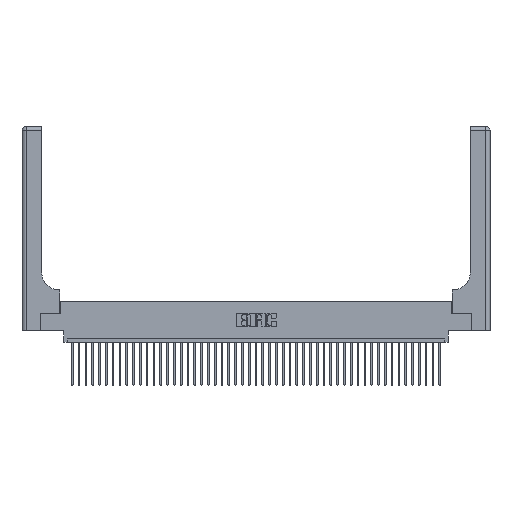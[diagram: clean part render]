
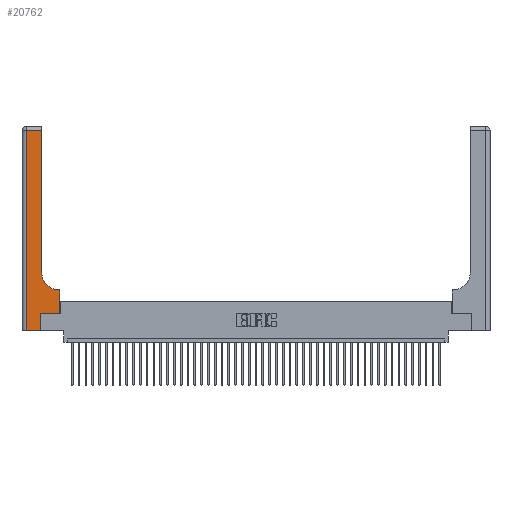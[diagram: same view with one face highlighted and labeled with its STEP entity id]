
A CAD part, top view. The second image highlights one B-rep face of the part: STEP entity #20762.
In plain terms, the highlighted planar face has unit normal (0, 0, 1).
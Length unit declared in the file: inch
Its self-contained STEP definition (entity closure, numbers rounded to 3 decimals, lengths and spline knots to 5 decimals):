
#450 = CARTESIAN_POINT ( 'NONE',  ( 0.269, 0.25, 0.37 ) ) ;
#1973 = VECTOR ( 'NONE', #14406, 39.37008 ) ;
#2352 = VERTEX_POINT ( 'NONE', #27724 ) ;
#2886 = ORIENTED_EDGE ( 'NONE', *, *, #30158, .T. ) ;
#3375 = CARTESIAN_POINT ( 'NONE',  ( 0.269, 0.25, 0.37 ) ) ;
#3590 = ORIENTED_EDGE ( 'NONE', *, *, #39294, .T. ) ;
#4475 = VERTEX_POINT ( 'NONE', #3375 ) ;
#4817 = ORIENTED_EDGE ( 'NONE', *, *, #18907, .T. ) ;
#7605 = ORIENTED_EDGE ( 'NONE', *, *, #14919, .T. ) ;
#8180 = CARTESIAN_POINT ( 'NONE',  ( 0.06, 3., 0.37 ) ) ;
#8871 = LINE ( 'NONE', #34067, #25203 ) ;
#9090 = DIRECTION ( 'NONE',  ( 0., 0., -1. ) ) ;
#10921 = CARTESIAN_POINT ( 'NONE',  ( 0., 2.94, 0.37 ) ) ;
#11401 = PLANE ( 'NONE',  #24227 ) ;
#11439 = CARTESIAN_POINT ( 'NONE',  ( 0.269, 0., 0.37 ) ) ;
#11601 = DIRECTION ( 'NONE',  ( 0., 1., 0. ) ) ;
#11639 = CARTESIAN_POINT ( 'NONE',  ( 0.5585, 0.6, 0.37 ) ) ;
#11847 = LINE ( 'NONE', #8180, #20040 ) ;
#14406 = DIRECTION ( 'NONE',  ( -1., 0., 0. ) ) ;
#14919 = EDGE_CURVE ( 'NONE', #36600, #4475, #21416, .T. ) ;
#17676 = DIRECTION ( 'NONE',  ( 1., 0., 0. ) ) ;
#18052 = LINE ( 'NONE', #23806, #31091 ) ;
#18601 = VECTOR ( 'NONE', #17676, 39.37008 ) ;
#18907 = EDGE_CURVE ( 'NONE', #31382, #20105, #8871, .T. ) ;
#19266 = EDGE_CURVE ( 'NONE', #42199, #25814, #41284, .T. ) ;
#19396 = FACE_OUTER_BOUND ( 'NONE', #33788, .T. ) ;
#19474 = CARTESIAN_POINT ( 'NONE',  ( 0.5415, 0.85, 0.37 ) ) ;
#20040 = VECTOR ( 'NONE', #28888, 39.37008 ) ;
#20105 = VERTEX_POINT ( 'NONE', #21958 ) ;
#20762 = ADVANCED_FACE ( 'NONE', ( #19396 ), #11401, .F. ) ;
#21416 = LINE ( 'NONE', #11439, #32293 ) ;
#21958 = CARTESIAN_POINT ( 'NONE',  ( 0.5415, 0.6, 0.37 ) ) ;
#22976 = DIRECTION ( 'NONE',  ( 1., 0., 0. ) ) ;
#23009 = LINE ( 'NONE', #40666, #27362 ) ;
#23417 = ORIENTED_EDGE ( 'NONE', *, *, #23950, .T. ) ;
#23806 = CARTESIAN_POINT ( 'NONE',  ( 0., 0., 0.37 ) ) ;
#23950 = EDGE_CURVE ( 'NONE', #44852, #36600, #18052, .T. ) ;
#24060 = LINE ( 'NONE', #450, #18601 ) ;
#24227 = AXIS2_PLACEMENT_3D ( 'NONE', #35729, #26311, #39600 ) ;
#25203 = VECTOR ( 'NONE', #27735, 39.37008 ) ;
#25814 = VERTEX_POINT ( 'NONE', #38619 ) ;
#26118 = CARTESIAN_POINT ( 'NONE',  ( 0.2915, 3., 0.37 ) ) ;
#26311 = DIRECTION ( 'NONE',  ( 0., 0., -1. ) ) ;
#27033 = CARTESIAN_POINT ( 'NONE',  ( 0.5585, 0.25, 0.37 ) ) ;
#27362 = VECTOR ( 'NONE', #33585, 39.37008 ) ;
#27724 = CARTESIAN_POINT ( 'NONE',  ( 0.06, 2.94, 0.37 ) ) ;
#27735 = DIRECTION ( 'NONE',  ( -1., 0., 0. ) ) ;
#28389 = ORIENTED_EDGE ( 'NONE', *, *, #41217, .T. ) ;
#28888 = DIRECTION ( 'NONE',  ( 0., -1., 0. ) ) ;
#29756 = CARTESIAN_POINT ( 'NONE',  ( 0.2915, 0.85, 0.37 ) ) ;
#30158 = EDGE_CURVE ( 'NONE', #20105, #42199, #40556, .T. ) ;
#30930 = DIRECTION ( 'NONE',  ( 1., 0., 0. ) ) ;
#31091 = VECTOR ( 'NONE', #30930, 39.37008 ) ;
#31382 = VERTEX_POINT ( 'NONE', #11639 ) ;
#31995 = AXIS2_PLACEMENT_3D ( 'NONE', #19474, #9090, #22976 ) ;
#32048 = ORIENTED_EDGE ( 'NONE', *, *, #41906, .T. ) ;
#32293 = VECTOR ( 'NONE', #11601, 39.37008 ) ;
#33358 = VERTEX_POINT ( 'NONE', #27033 ) ;
#33585 = DIRECTION ( 'NONE',  ( 0., 1., 0. ) ) ;
#33788 = EDGE_LOOP ( 'NONE', ( #38550, #32048, #28389, #23417, #7605, #3590, #41645, #4817, #2886 ) ) ;
#34067 = CARTESIAN_POINT ( 'NONE',  ( 0.2915, 0.6, 0.37 ) ) ;
#35729 = CARTESIAN_POINT ( 'NONE',  ( 0., 3., 0.37 ) ) ;
#36198 = CARTESIAN_POINT ( 'NONE',  ( 0.269, 0., 0.37 ) ) ;
#36600 = VERTEX_POINT ( 'NONE', #36198 ) ;
#36790 = LINE ( 'NONE', #10921, #1973 ) ;
#37755 = CARTESIAN_POINT ( 'NONE',  ( 0.06, 0., 0.37 ) ) ;
#38452 = EDGE_CURVE ( 'NONE', #33358, #31382, #23009, .T. ) ;
#38550 = ORIENTED_EDGE ( 'NONE', *, *, #19266, .T. ) ;
#38619 = CARTESIAN_POINT ( 'NONE',  ( 0.2915, 2.94, 0.37 ) ) ;
#39070 = VECTOR ( 'NONE', #39586, 39.37008 ) ;
#39294 = EDGE_CURVE ( 'NONE', #4475, #33358, #24060, .T. ) ;
#39586 = DIRECTION ( 'NONE',  ( 0., 1., 0. ) ) ;
#39600 = DIRECTION ( 'NONE',  ( -1., 0., 0. ) ) ;
#40556 = CIRCLE ( 'NONE', #31995, 0.25 ) ;
#40666 = CARTESIAN_POINT ( 'NONE',  ( 0.5585, 0.25, 0.37 ) ) ;
#41217 = EDGE_CURVE ( 'NONE', #2352, #44852, #11847, .T. ) ;
#41284 = LINE ( 'NONE', #26118, #39070 ) ;
#41645 = ORIENTED_EDGE ( 'NONE', *, *, #38452, .T. ) ;
#41906 = EDGE_CURVE ( 'NONE', #25814, #2352, #36790, .T. ) ;
#42199 = VERTEX_POINT ( 'NONE', #29756 ) ;
#44852 = VERTEX_POINT ( 'NONE', #37755 ) ;
